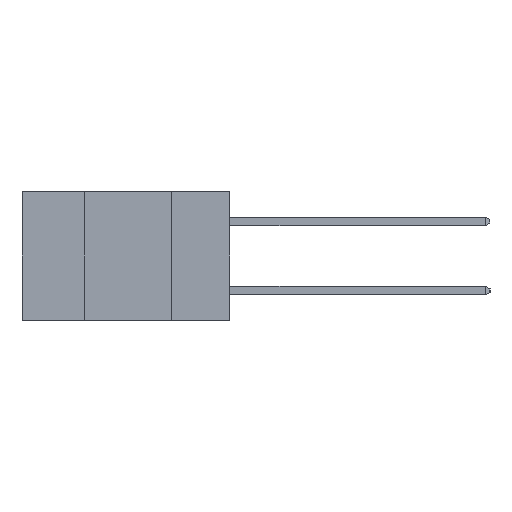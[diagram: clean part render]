
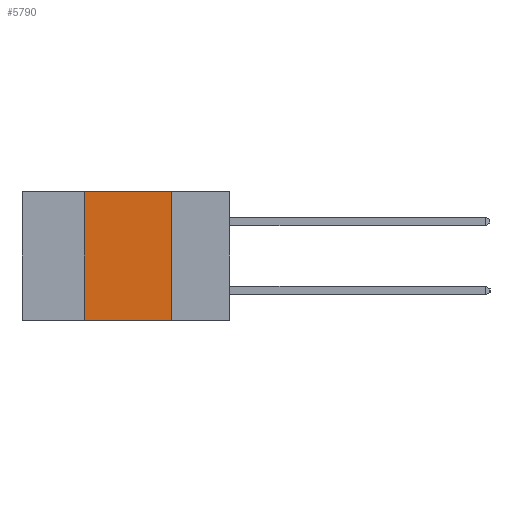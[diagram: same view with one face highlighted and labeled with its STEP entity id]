
A CAD part, left-side view. The second image highlights one B-rep face of the part: STEP entity #5790.
In plain terms, the highlighted planar face has unit normal (-1, 0, 0).
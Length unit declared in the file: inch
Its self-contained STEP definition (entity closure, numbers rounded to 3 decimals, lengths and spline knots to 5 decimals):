
#166 = EDGE_CURVE ( 'NONE', #6267, #7168, #12769, .T. ) ;
#576 = PLANE ( 'NONE',  #13926 ) ;
#1151 = CARTESIAN_POINT ( 'NONE',  ( 0., 0.42, -0.37 ) ) ;
#1214 = VERTEX_POINT ( 'NONE', #8357 ) ;
#1604 = EDGE_LOOP ( 'NONE', ( #6981, #7332, #12963, #1626 ) ) ;
#1626 = ORIENTED_EDGE ( 'NONE', *, *, #11074, .T. ) ;
#3797 = DIRECTION ( 'NONE',  ( 0., -1., 0. ) ) ;
#3832 = DIRECTION ( 'NONE',  ( 0., 0., -1. ) ) ;
#4188 = FACE_OUTER_BOUND ( 'NONE', #1604, .T. ) ;
#4388 = CARTESIAN_POINT ( 'NONE',  ( 0., 0.6, -0.37 ) ) ;
#5781 = LINE ( 'NONE', #1151, #11225 ) ;
#5790 = ADVANCED_FACE ( 'NONE', ( #4188 ), #576, .F. ) ;
#6267 = VERTEX_POINT ( 'NONE', #10937 ) ;
#6868 = LINE ( 'NONE', #4388, #9098 ) ;
#6981 = ORIENTED_EDGE ( 'NONE', *, *, #12129, .F. ) ;
#7168 = VERTEX_POINT ( 'NONE', #7613 ) ;
#7332 = ORIENTED_EDGE ( 'NONE', *, *, #166, .F. ) ;
#7613 = CARTESIAN_POINT ( 'NONE',  ( 0., 0.17, 0. ) ) ;
#8357 = CARTESIAN_POINT ( 'NONE',  ( 0., 0.17, -0.37 ) ) ;
#9098 = VECTOR ( 'NONE', #3797, 39.37008 ) ;
#9422 = DIRECTION ( 'NONE',  ( 0., -1., 0. ) ) ;
#9541 = VECTOR ( 'NONE', #3832, 39.37008 ) ;
#9979 = VECTOR ( 'NONE', #9422, 39.37008 ) ;
#10045 = CARTESIAN_POINT ( 'NONE',  ( 0., 0.6, 0. ) ) ;
#10078 = DIRECTION ( 'NONE',  ( 0., 0., 1. ) ) ;
#10937 = CARTESIAN_POINT ( 'NONE',  ( 0., 0.42, 0. ) ) ;
#11074 = EDGE_CURVE ( 'NONE', #13756, #1214, #6868, .T. ) ;
#11225 = VECTOR ( 'NONE', #10078, 39.37008 ) ;
#11503 = CARTESIAN_POINT ( 'NONE',  ( 0., 0.17, -0.37 ) ) ;
#11967 = CARTESIAN_POINT ( 'NONE',  ( 0., 0.42, -0.37 ) ) ;
#12129 = EDGE_CURVE ( 'NONE', #7168, #1214, #12361, .T. ) ;
#12361 = LINE ( 'NONE', #11503, #9541 ) ;
#12561 = EDGE_CURVE ( 'NONE', #13756, #6267, #5781, .T. ) ;
#12769 = LINE ( 'NONE', #10045, #9979 ) ;
#12963 = ORIENTED_EDGE ( 'NONE', *, *, #12561, .F. ) ;
#13756 = VERTEX_POINT ( 'NONE', #11967 ) ;
#13926 = AXIS2_PLACEMENT_3D ( 'NONE', #14075, #14012, #13980 ) ;
#13980 = DIRECTION ( 'NONE',  ( 0., 0., -1. ) ) ;
#14012 = DIRECTION ( 'NONE',  ( 1., 0., 0. ) ) ;
#14075 = CARTESIAN_POINT ( 'NONE',  ( 0., 0.6, 0. ) ) ;
